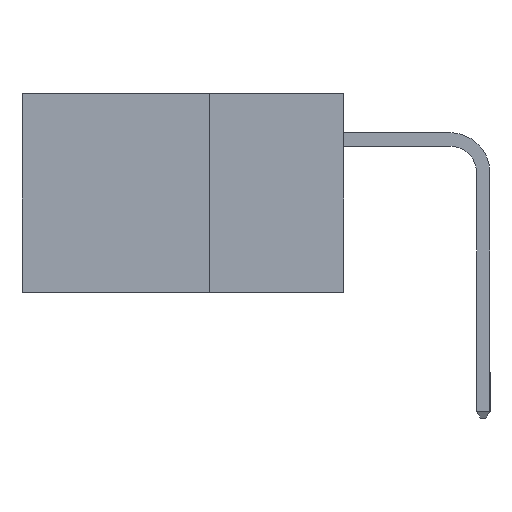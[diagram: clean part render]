
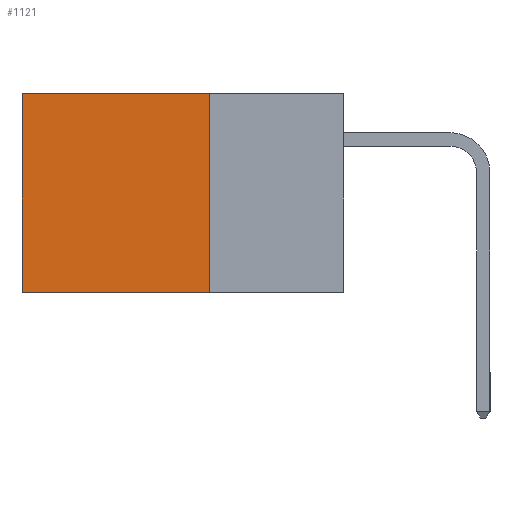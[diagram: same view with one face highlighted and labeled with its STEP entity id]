
A CAD part, left-side view. The second image highlights one B-rep face of the part: STEP entity #1121.
In plain terms, the highlighted planar face has unit normal (-1, 0, 0).
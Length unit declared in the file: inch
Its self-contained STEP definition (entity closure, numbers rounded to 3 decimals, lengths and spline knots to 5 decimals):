
#593 = VECTOR ( 'NONE', #5872, 39.37008 ) ;
#1014 = CARTESIAN_POINT ( 'NONE',  ( 0.298, 0.25, 0. ) ) ;
#1121 = ADVANCED_FACE ( 'NONE', ( #10697 ), #2623, .F. ) ;
#1504 = LINE ( 'NONE', #10504, #8804 ) ;
#1658 = LINE ( 'NONE', #12089, #11113 ) ;
#1942 = CARTESIAN_POINT ( 'NONE',  ( 0.298, 0.25, -0.37 ) ) ;
#2284 = CARTESIAN_POINT ( 'NONE',  ( 0.298, 0.25, -0.37 ) ) ;
#2623 = PLANE ( 'NONE',  #3030 ) ;
#2729 = ORIENTED_EDGE ( 'NONE', *, *, #7561, .F. ) ;
#2890 = LINE ( 'NONE', #8756, #9873 ) ;
#3030 = AXIS2_PLACEMENT_3D ( 'NONE', #7526, #5661, #12555 ) ;
#3318 = ORIENTED_EDGE ( 'NONE', *, *, #9724, .F. ) ;
#4078 = EDGE_CURVE ( 'NONE', #11595, #6599, #1504, .T. ) ;
#4576 = DIRECTION ( 'NONE',  ( 0., 0., -1. ) ) ;
#5098 = ORIENTED_EDGE ( 'NONE', *, *, #4078, .T. ) ;
#5244 = LINE ( 'NONE', #1942, #593 ) ;
#5661 = DIRECTION ( 'NONE',  ( 1., 0., 0. ) ) ;
#5872 = DIRECTION ( 'NONE',  ( 0., 1., 0. ) ) ;
#6599 = VERTEX_POINT ( 'NONE', #10555 ) ;
#6666 = ORIENTED_EDGE ( 'NONE', *, *, #7991, .T. ) ;
#6885 = VERTEX_POINT ( 'NONE', #2284 ) ;
#7526 = CARTESIAN_POINT ( 'NONE',  ( 0.298, 0.25, 0. ) ) ;
#7561 = EDGE_CURVE ( 'NONE', #6885, #6599, #5244, .T. ) ;
#7991 = EDGE_CURVE ( 'NONE', #12788, #11595, #1658, .T. ) ;
#8756 = CARTESIAN_POINT ( 'NONE',  ( 0.298, 0.25, 0. ) ) ;
#8804 = VECTOR ( 'NONE', #4576, 39.37008 ) ;
#9724 = EDGE_CURVE ( 'NONE', #12788, #6885, #2890, .T. ) ;
#9756 = DIRECTION ( 'NONE',  ( 0., 0., -1. ) ) ;
#9873 = VECTOR ( 'NONE', #9756, 39.37008 ) ;
#10450 = EDGE_LOOP ( 'NONE', ( #5098, #2729, #3318, #6666 ) ) ;
#10504 = CARTESIAN_POINT ( 'NONE',  ( 0.298, 0.6, 0. ) ) ;
#10555 = CARTESIAN_POINT ( 'NONE',  ( 0.298, 0.6, -0.37 ) ) ;
#10697 = FACE_OUTER_BOUND ( 'NONE', #10450, .T. ) ;
#11113 = VECTOR ( 'NONE', #12332, 39.37008 ) ;
#11595 = VERTEX_POINT ( 'NONE', #12617 ) ;
#12089 = CARTESIAN_POINT ( 'NONE',  ( 0.298, 0.25, 0. ) ) ;
#12332 = DIRECTION ( 'NONE',  ( 0., 1., 0. ) ) ;
#12555 = DIRECTION ( 'NONE',  ( 0., 0., -1. ) ) ;
#12617 = CARTESIAN_POINT ( 'NONE',  ( 0.298, 0.6, 0. ) ) ;
#12788 = VERTEX_POINT ( 'NONE', #1014 ) ;
